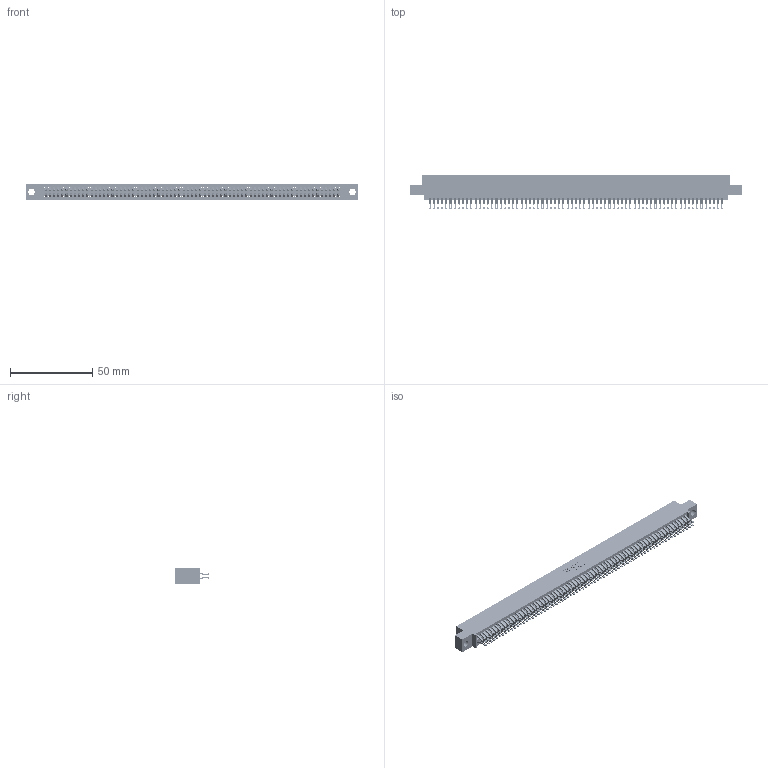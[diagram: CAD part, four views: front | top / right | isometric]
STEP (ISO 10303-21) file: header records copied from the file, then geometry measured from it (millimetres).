
FILE_DESCRIPTION (( 'STEP AP203' ), '1' );
FILE_NAME ('395-142-555-504.STEP', '2021-06-18T05:37:15', ( '' ), ( '' ), 'SwSTEP 2.0', 'SolidWorks 2020', '' );
FILE_SCHEMA (( 'CONFIG_CONTROL_DESIGN' ));
Length unit declared in the file: inch
Products named in the file (3): 345-292-001_555 Tail; 395-142-555-504; 345 Part_0.110 Offset - 0.156 Dia-TI
Assembly tree (143 placements, depth 2):
  395-142-555-504
    345 Part_0.110 Offset - 0.156 Dia-TI
    345-292-001_555 Tail  x142
Bounding box: 201.55 x 21.13 x 9.4 mm (x, y, z)
Volume: 20080.4 mm3; surface area: 31620.9 mm2
Topology: 143 solids, 143 shells, 8096 faces, 25523 edges, 17014 vertices
Faces by surface type: plane 4500, cylinder 3596
Entity records: 52681 total; most frequent: CARTESIAN_POINT 8844, ORIENTED_EDGE 8746, DIRECTION 7729, EDGE_CURVE 4373, VECTOR 3937, LINE 3937, VERTEX_POINT 2914, AXIS2_PLACEMENT_3D 1896
